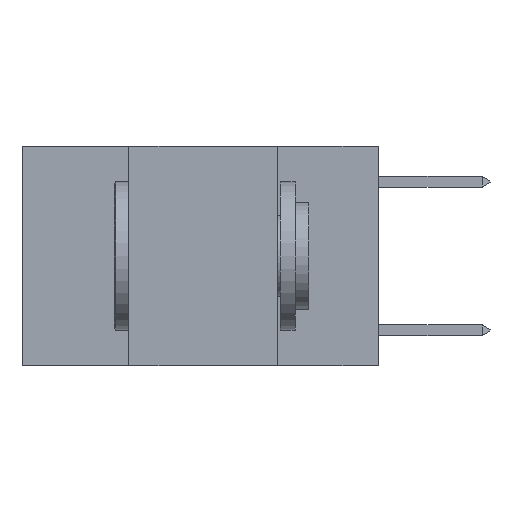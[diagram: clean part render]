
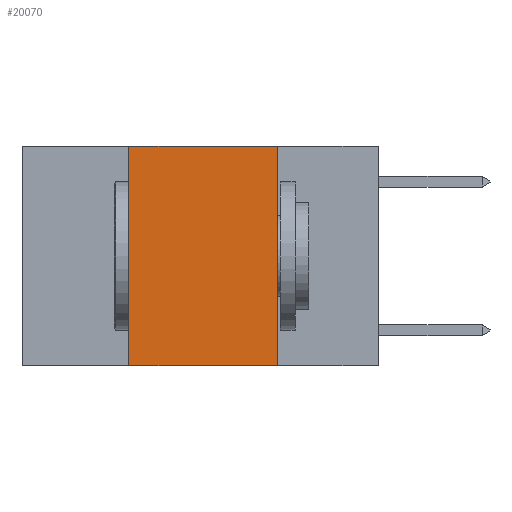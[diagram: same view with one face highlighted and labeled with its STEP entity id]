
A CAD part, left-side view. The second image highlights one B-rep face of the part: STEP entity #20070.
In plain terms, the highlighted planar face has unit normal (-1, 0, 0).
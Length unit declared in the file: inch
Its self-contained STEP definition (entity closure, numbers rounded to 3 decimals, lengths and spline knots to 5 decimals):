
#1334 = VERTEX_POINT ( 'NONE', #14110 ) ;
#1421 = FACE_OUTER_BOUND ( 'NONE', #21337, .T. ) ;
#3492 = VECTOR ( 'NONE', #14722, 39.37008 ) ;
#3543 = CARTESIAN_POINT ( 'NONE',  ( 0., 0.17, -0.37 ) ) ;
#4324 = VERTEX_POINT ( 'NONE', #3543 ) ;
#5080 = EDGE_CURVE ( 'NONE', #16690, #1334, #15506, .T. ) ;
#5139 = PLANE ( 'NONE',  #6931 ) ;
#6160 = LINE ( 'NONE', #11039, #15075 ) ;
#6405 = EDGE_CURVE ( 'NONE', #16690, #4324, #18345, .T. ) ;
#6931 = AXIS2_PLACEMENT_3D ( 'NONE', #13663, #8518, #15542 ) ;
#8370 = DIRECTION ( 'NONE',  ( 0., 0., 1. ) ) ;
#8518 = DIRECTION ( 'NONE',  ( 1., 0., 0. ) ) ;
#9552 = VECTOR ( 'NONE', #11274, 39.37008 ) ;
#9576 = VECTOR ( 'NONE', #8370, 39.37008 ) ;
#11039 = CARTESIAN_POINT ( 'NONE',  ( 0., 0.6, 0. ) ) ;
#11130 = CARTESIAN_POINT ( 'NONE',  ( 0., 0.42, -0.37 ) ) ;
#11274 = DIRECTION ( 'NONE',  ( 0., 0., -1. ) ) ;
#11393 = CARTESIAN_POINT ( 'NONE',  ( 0., 0.17, 0. ) ) ;
#11546 = CARTESIAN_POINT ( 'NONE',  ( 0., 0.6, -0.37 ) ) ;
#13272 = DIRECTION ( 'NONE',  ( 0., -1., 0. ) ) ;
#13663 = CARTESIAN_POINT ( 'NONE',  ( 0., 0.6, 0. ) ) ;
#13733 = ORIENTED_EDGE ( 'NONE', *, *, #5080, .F. ) ;
#13734 = CARTESIAN_POINT ( 'NONE',  ( 0., 0.42, 0. ) ) ;
#14110 = CARTESIAN_POINT ( 'NONE',  ( 0., 0.42, 0. ) ) ;
#14722 = DIRECTION ( 'NONE',  ( 0., -1., 0. ) ) ;
#15075 = VECTOR ( 'NONE', #13272, 39.37008 ) ;
#15457 = CARTESIAN_POINT ( 'NONE',  ( 0., 0.17, 0. ) ) ;
#15506 = LINE ( 'NONE', #13734, #9576 ) ;
#15542 = DIRECTION ( 'NONE',  ( 0., 0., -1. ) ) ;
#16351 = EDGE_CURVE ( 'NONE', #1334, #21225, #6160, .T. ) ;
#16690 = VERTEX_POINT ( 'NONE', #11130 ) ;
#17302 = ORIENTED_EDGE ( 'NONE', *, *, #16351, .F. ) ;
#17471 = ORIENTED_EDGE ( 'NONE', *, *, #20809, .F. ) ;
#18345 = LINE ( 'NONE', #11546, #3492 ) ;
#19650 = ORIENTED_EDGE ( 'NONE', *, *, #6405, .T. ) ;
#20070 = ADVANCED_FACE ( 'NONE', ( #1421 ), #5139, .F. ) ;
#20172 = LINE ( 'NONE', #11393, #9552 ) ;
#20809 = EDGE_CURVE ( 'NONE', #21225, #4324, #20172, .T. ) ;
#21225 = VERTEX_POINT ( 'NONE', #15457 ) ;
#21337 = EDGE_LOOP ( 'NONE', ( #17471, #17302, #13733, #19650 ) ) ;
